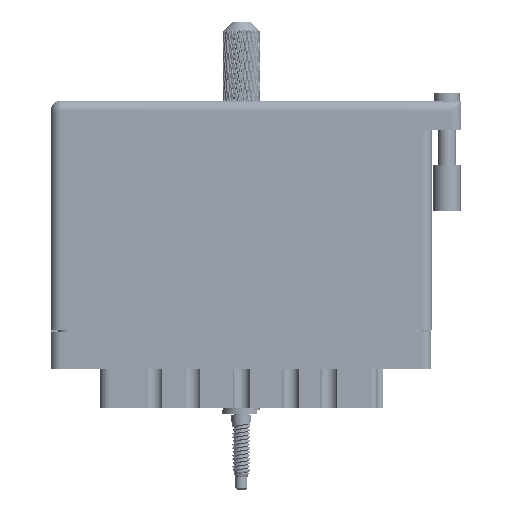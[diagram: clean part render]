
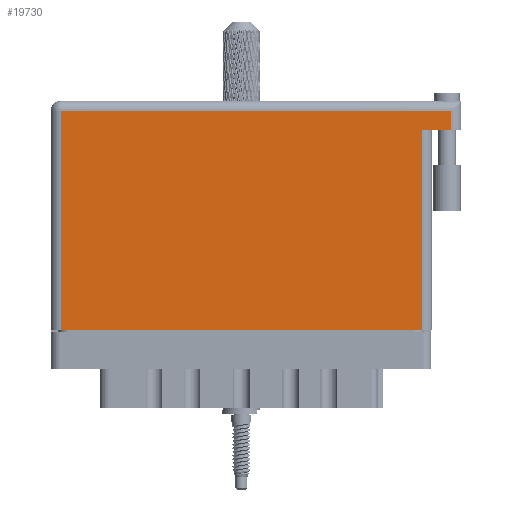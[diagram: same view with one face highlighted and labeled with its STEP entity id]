
A CAD part, front view. The second image highlights one B-rep face of the part: STEP entity #19730.
In plain terms, the highlighted face is planar.
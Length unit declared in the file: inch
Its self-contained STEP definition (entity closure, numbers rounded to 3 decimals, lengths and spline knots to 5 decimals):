
#2694 = EDGE_CURVE ( 'NONE', #10458, #61639, #108142, .T. ) ;
#3375 = CARTESIAN_POINT ( 'NONE',  ( 2.8, 1.369, 0. ) ) ;
#3864 = DIRECTION ( 'NONE',  ( -1., 0., 0. ) ) ;
#7497 = CARTESIAN_POINT ( 'NONE',  ( 0.07, 1.496, 0. ) ) ;
#8863 = LINE ( 'NONE', #111782, #105224 ) ;
#10458 = VERTEX_POINT ( 'NONE', #39870 ) ;
#12651 = DIRECTION ( 'NONE',  ( -1., 0., 0. ) ) ;
#15837 = EDGE_LOOP ( 'NONE', ( #73805, #37321, #35705, #44747, #87574, #98391 ) ) ;
#19730 = ADVANCED_FACE ( 'NONE', ( #24143 ), #31564, .F. ) ;
#20702 = CARTESIAN_POINT ( 'NONE',  ( 2.53, 1.369, 0. ) ) ;
#24143 = FACE_OUTER_BOUND ( 'NONE', #15837, .T. ) ;
#27698 = EDGE_CURVE ( 'NONE', #54211, #61639, #34773, .T. ) ;
#31564 = PLANE ( 'NONE',  #61721 ) ;
#33078 = VERTEX_POINT ( 'NONE', #94159 ) ;
#34761 = VECTOR ( 'NONE', #38303, 39.37008 ) ;
#34773 = LINE ( 'NONE', #3375, #92349 ) ;
#35705 = ORIENTED_EDGE ( 'NONE', *, *, #27698, .F. ) ;
#37075 = LINE ( 'NONE', #46059, #67290 ) ;
#37321 = ORIENTED_EDGE ( 'NONE', *, *, #2694, .T. ) ;
#38303 = DIRECTION ( 'NONE',  ( 0., 1., 0. ) ) ;
#38711 = DIRECTION ( 'NONE',  ( 1., 0., 0. ) ) ;
#39870 = CARTESIAN_POINT ( 'NONE',  ( 2.53, 0., 0. ) ) ;
#40837 = CARTESIAN_POINT ( 'NONE',  ( 0., 1.566, 0. ) ) ;
#44747 = ORIENTED_EDGE ( 'NONE', *, *, #70852, .T. ) ;
#46059 = CARTESIAN_POINT ( 'NONE',  ( 0., 1.496, 0. ) ) ;
#49673 = DIRECTION ( 'NONE',  ( 0., 0., -1. ) ) ;
#54211 = VERTEX_POINT ( 'NONE', #81687 ) ;
#56755 = DIRECTION ( 'NONE',  ( 0., 1., 0. ) ) ;
#56876 = CARTESIAN_POINT ( 'NONE',  ( 2.53, 1.369, 0. ) ) ;
#61639 = VERTEX_POINT ( 'NONE', #20702 ) ;
#61721 = AXIS2_PLACEMENT_3D ( 'NONE', #40837, #49673, #3864 ) ;
#63465 = CARTESIAN_POINT ( 'NONE',  ( 0.07, 0., 0. ) ) ;
#63809 = DIRECTION ( 'NONE',  ( -1., 0., 0. ) ) ;
#64521 = EDGE_CURVE ( 'NONE', #90552, #10458, #77552, .T. ) ;
#67290 = VECTOR ( 'NONE', #63809, 39.37008 ) ;
#70852 = EDGE_CURVE ( 'NONE', #54211, #33078, #8863, .T. ) ;
#73805 = ORIENTED_EDGE ( 'NONE', *, *, #64521, .T. ) ;
#76712 = VERTEX_POINT ( 'NONE', #7497 ) ;
#77552 = LINE ( 'NONE', #102622, #83295 ) ;
#81476 = DIRECTION ( 'NONE',  ( 0., -1., 0. ) ) ;
#81687 = CARTESIAN_POINT ( 'NONE',  ( 2.73, 1.369, 0. ) ) ;
#83295 = VECTOR ( 'NONE', #38711, 39.37008 ) ;
#87574 = ORIENTED_EDGE ( 'NONE', *, *, #113927, .T. ) ;
#88517 = LINE ( 'NONE', #63465, #114430 ) ;
#90552 = VERTEX_POINT ( 'NONE', #110555 ) ;
#92349 = VECTOR ( 'NONE', #12651, 39.37008 ) ;
#94159 = CARTESIAN_POINT ( 'NONE',  ( 2.73, 1.496, 0. ) ) ;
#98391 = ORIENTED_EDGE ( 'NONE', *, *, #116103, .T. ) ;
#102622 = CARTESIAN_POINT ( 'NONE',  ( 0., 0., 0. ) ) ;
#105224 = VECTOR ( 'NONE', #56755, 39.37008 ) ;
#108142 = LINE ( 'NONE', #56876, #34761 ) ;
#110555 = CARTESIAN_POINT ( 'NONE',  ( 0.07, 0., 0. ) ) ;
#111782 = CARTESIAN_POINT ( 'NONE',  ( 2.73, 1.566, 0. ) ) ;
#113927 = EDGE_CURVE ( 'NONE', #33078, #76712, #37075, .T. ) ;
#114430 = VECTOR ( 'NONE', #81476, 39.37008 ) ;
#116103 = EDGE_CURVE ( 'NONE', #76712, #90552, #88517, .T. ) ;
